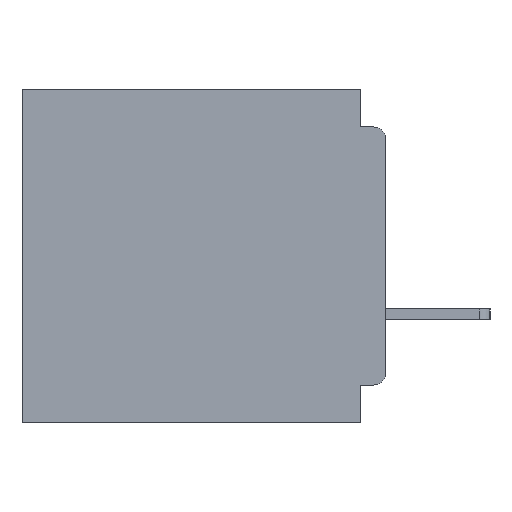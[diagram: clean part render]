
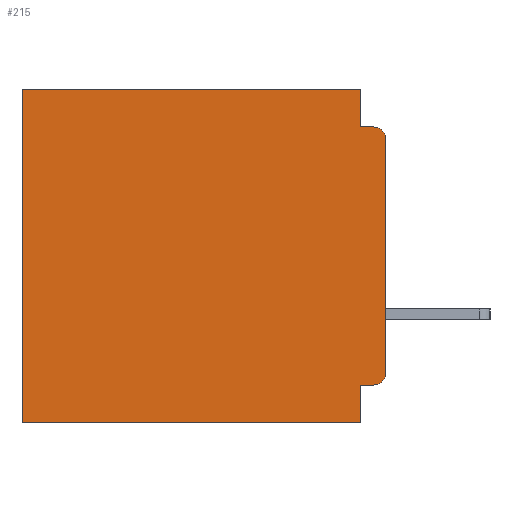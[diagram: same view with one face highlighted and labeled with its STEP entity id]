
A CAD part, left-side view. The second image highlights one B-rep face of the part: STEP entity #215.
In plain terms, the highlighted planar face has unit normal (-1, 0, 0).
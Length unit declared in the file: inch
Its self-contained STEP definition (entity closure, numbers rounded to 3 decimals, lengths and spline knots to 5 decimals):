
#147 = CARTESIAN_POINT ( 'NONE',  ( 0.3, 0., -0.4 ) ) ;
#215 = ADVANCED_FACE ( 'NONE', ( #43387 ), #1419, .F. ) ;
#1311 = ORIENTED_EDGE ( 'NONE', *, *, #11445, .T. ) ;
#1419 = PLANE ( 'NONE',  #38507 ) ;
#1440 = CARTESIAN_POINT ( 'NONE',  ( 0.3, 0.031, -0.4 ) ) ;
#1717 = EDGE_CURVE ( 'NONE', #31796, #57345, #57870, .T. ) ;
#3131 = DIRECTION ( 'NONE',  ( 0., 0., -1. ) ) ;
#3313 = CARTESIAN_POINT ( 'NONE',  ( 0.3, 0.031, -0.355 ) ) ;
#4038 = CARTESIAN_POINT ( 'NONE',  ( 0.3, 0., 0. ) ) ;
#7445 = DIRECTION ( 'NONE',  ( -1., 0., 0. ) ) ;
#8919 = VECTOR ( 'NONE', #47906, 39.37008 ) ;
#8999 = LINE ( 'NONE', #24891, #32449 ) ;
#9002 = EDGE_CURVE ( 'NONE', #49726, #48648, #46238, .T. ) ;
#11445 = EDGE_CURVE ( 'NONE', #23440, #25919, #35591, .T. ) ;
#12557 = CARTESIAN_POINT ( 'NONE',  ( 0.3, 0.031, -0.4 ) ) ;
#13215 = VERTEX_POINT ( 'NONE', #16626 ) ;
#13891 = ORIENTED_EDGE ( 'NONE', *, *, #44133, .F. ) ;
#14920 = DIRECTION ( 'NONE',  ( 0., 1., 0. ) ) ;
#16626 = CARTESIAN_POINT ( 'NONE',  ( 0.3, 0.015, -0.045 ) ) ;
#17399 = ORIENTED_EDGE ( 'NONE', *, *, #37784, .F. ) ;
#17453 = ORIENTED_EDGE ( 'NONE', *, *, #57166, .T. ) ;
#17927 = CARTESIAN_POINT ( 'NONE',  ( 0.3, 0., -0.06 ) ) ;
#17985 = CARTESIAN_POINT ( 'NONE',  ( 0.3, 0.031, 0. ) ) ;
#17999 = DIRECTION ( 'NONE',  ( 0., 0., -1. ) ) ;
#19291 = ORIENTED_EDGE ( 'NONE', *, *, #46560, .F. ) ;
#19682 = VERTEX_POINT ( 'NONE', #17927 ) ;
#22264 = CIRCLE ( 'NONE', #44891, 0.015 ) ;
#22767 = CARTESIAN_POINT ( 'NONE',  ( 0.3, 0., -0.4 ) ) ;
#23440 = VERTEX_POINT ( 'NONE', #17985 ) ;
#24891 = CARTESIAN_POINT ( 'NONE',  ( 0.3, 0., -0.4 ) ) ;
#25329 = DIRECTION ( 'NONE',  ( -1., 0., 0. ) ) ;
#25919 = VERTEX_POINT ( 'NONE', #28007 ) ;
#26874 = LINE ( 'NONE', #57590, #51698 ) ;
#28007 = CARTESIAN_POINT ( 'NONE',  ( 0.3, 0.437, 0. ) ) ;
#28582 = CIRCLE ( 'NONE', #34841, 0.015 ) ;
#28848 = EDGE_CURVE ( 'NONE', #25919, #57345, #47874, .T. ) ;
#29569 = DIRECTION ( 'NONE',  ( 0., -1., 0. ) ) ;
#30196 = DIRECTION ( 'NONE',  ( 1., 0., 0. ) ) ;
#31334 = EDGE_CURVE ( 'NONE', #19682, #13215, #28582, .T. ) ;
#31796 = VERTEX_POINT ( 'NONE', #1440 ) ;
#31956 = ORIENTED_EDGE ( 'NONE', *, *, #31334, .T. ) ;
#32449 = VECTOR ( 'NONE', #43434, 39.37008 ) ;
#33644 = VERTEX_POINT ( 'NONE', #40532 ) ;
#34841 = AXIS2_PLACEMENT_3D ( 'NONE', #35482, #7445, #40185 ) ;
#35470 = VECTOR ( 'NONE', #17999, 39.37008 ) ;
#35482 = CARTESIAN_POINT ( 'NONE',  ( 0.3, 0.015, -0.06 ) ) ;
#35516 = VECTOR ( 'NONE', #40527, 39.37008 ) ;
#35591 = LINE ( 'NONE', #4038, #38542 ) ;
#36556 = CARTESIAN_POINT ( 'NONE',  ( 0.3, 0.437, -0.4 ) ) ;
#36797 = DIRECTION ( 'NONE',  ( 0., 1., 0. ) ) ;
#37439 = DIRECTION ( 'NONE',  ( 0., 0., -1. ) ) ;
#37784 = EDGE_CURVE ( 'NONE', #55870, #13215, #26874, .T. ) ;
#38477 = LINE ( 'NONE', #12557, #35516 ) ;
#38507 = AXIS2_PLACEMENT_3D ( 'NONE', #22767, #30196, #3131 ) ;
#38542 = VECTOR ( 'NONE', #36797, 39.37008 ) ;
#39464 = ORIENTED_EDGE ( 'NONE', *, *, #1717, .F. ) ;
#40185 = DIRECTION ( 'NONE',  ( 0., 0., -1. ) ) ;
#40527 = DIRECTION ( 'NONE',  ( 0., 0., -1. ) ) ;
#40532 = CARTESIAN_POINT ( 'NONE',  ( 0.3, 0., -0.34 ) ) ;
#42274 = VECTOR ( 'NONE', #37439, 39.37008 ) ;
#43249 = CARTESIAN_POINT ( 'NONE',  ( 0.3, 0., -0.355 ) ) ;
#43387 = FACE_OUTER_BOUND ( 'NONE', #59675, .T. ) ;
#43434 = DIRECTION ( 'NONE',  ( 0., 0., -1. ) ) ;
#43750 = LINE ( 'NONE', #51351, #42274 ) ;
#44133 = EDGE_CURVE ( 'NONE', #23440, #55870, #43750, .T. ) ;
#44891 = AXIS2_PLACEMENT_3D ( 'NONE', #53293, #25329, #58025 ) ;
#46238 = LINE ( 'NONE', #43249, #8919 ) ;
#46560 = EDGE_CURVE ( 'NONE', #19682, #33644, #8999, .T. ) ;
#47874 = LINE ( 'NONE', #36556, #35470 ) ;
#47906 = DIRECTION ( 'NONE',  ( 0., 1., 0. ) ) ;
#48304 = CARTESIAN_POINT ( 'NONE',  ( 0.3, 0.031, -0.045 ) ) ;
#48648 = VERTEX_POINT ( 'NONE', #3313 ) ;
#49226 = ORIENTED_EDGE ( 'NONE', *, *, #28848, .T. ) ;
#49726 = VERTEX_POINT ( 'NONE', #56699 ) ;
#51351 = CARTESIAN_POINT ( 'NONE',  ( 0.3, 0.031, 0. ) ) ;
#51446 = ORIENTED_EDGE ( 'NONE', *, *, #56055, .F. ) ;
#51698 = VECTOR ( 'NONE', #29569, 39.37008 ) ;
#53293 = CARTESIAN_POINT ( 'NONE',  ( 0.3, 0.015, -0.34 ) ) ;
#54153 = ORIENTED_EDGE ( 'NONE', *, *, #9002, .F. ) ;
#54508 = CARTESIAN_POINT ( 'NONE',  ( 0.3, 0.437, -0.4 ) ) ;
#55870 = VERTEX_POINT ( 'NONE', #48304 ) ;
#56055 = EDGE_CURVE ( 'NONE', #48648, #31796, #38477, .T. ) ;
#56384 = VECTOR ( 'NONE', #14920, 39.37008 ) ;
#56699 = CARTESIAN_POINT ( 'NONE',  ( 0.3, 0.015, -0.355 ) ) ;
#57166 = EDGE_CURVE ( 'NONE', #49726, #33644, #22264, .T. ) ;
#57345 = VERTEX_POINT ( 'NONE', #54508 ) ;
#57590 = CARTESIAN_POINT ( 'NONE',  ( 0.3, 0., -0.045 ) ) ;
#57870 = LINE ( 'NONE', #147, #56384 ) ;
#58025 = DIRECTION ( 'NONE',  ( 0., 0., -1. ) ) ;
#59675 = EDGE_LOOP ( 'NONE', ( #19291, #31956, #17399, #13891, #1311, #49226, #39464, #51446, #54153, #17453 ) ) ;
